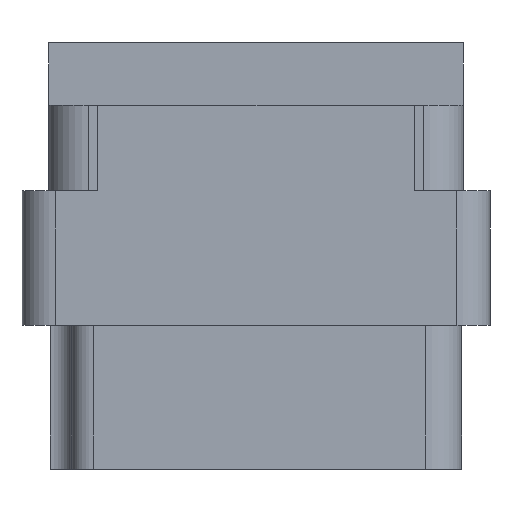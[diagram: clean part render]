
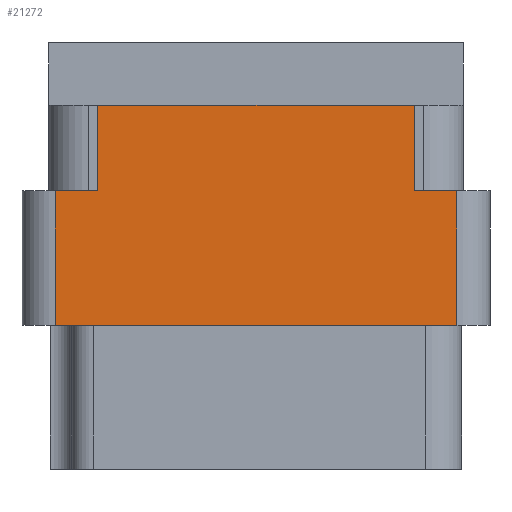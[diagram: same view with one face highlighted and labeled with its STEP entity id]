
A CAD part, left-side view. The second image highlights one B-rep face of the part: STEP entity #21272.
In plain terms, the highlighted planar face has unit normal (-1, 0, 0).
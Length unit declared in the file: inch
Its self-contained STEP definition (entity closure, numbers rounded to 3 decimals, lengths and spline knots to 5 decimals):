
#148 = LINE ( 'NONE', #6641, #24784 ) ;
#484 = CARTESIAN_POINT ( 'NONE',  ( -1., -0.296, -0.277 ) ) ;
#1525 = LINE ( 'NONE', #2006, #23892 ) ;
#2006 = CARTESIAN_POINT ( 'NONE',  ( -1., 0.376, -0.798 ) ) ;
#3123 = VECTOR ( 'NONE', #9455, 39.37008 ) ;
#3602 = ORIENTED_EDGE ( 'NONE', *, *, #24402, .T. ) ;
#3899 = CARTESIAN_POINT ( 'NONE',  ( -1., 0.438, -0.117 ) ) ;
#4356 = VERTEX_POINT ( 'NONE', #29186 ) ;
#5796 = LINE ( 'NONE', #8620, #27107 ) ;
#6131 = FACE_OUTER_BOUND ( 'NONE', #24997, .T. ) ;
#6449 = DIRECTION ( 'NONE',  ( 0., -1., 0. ) ) ;
#6541 = ORIENTED_EDGE ( 'NONE', *, *, #11253, .F. ) ;
#6623 = DIRECTION ( 'NONE',  ( 0., -1., 0. ) ) ;
#6641 = CARTESIAN_POINT ( 'NONE',  ( -1., 0., -0.277 ) ) ;
#6715 = EDGE_CURVE ( 'NONE', #22369, #12009, #7231, .T. ) ;
#6824 = DIRECTION ( 'NONE',  ( -1., 0., 0. ) ) ;
#7122 = VECTOR ( 'NONE', #14077, 39.37008 ) ;
#7231 = LINE ( 'NONE', #28528, #3123 ) ;
#8423 = CARTESIAN_POINT ( 'NONE',  ( -1., 0.376, -0.277 ) ) ;
#8446 = ORIENTED_EDGE ( 'NONE', *, *, #28309, .F. ) ;
#8620 = CARTESIAN_POINT ( 'NONE',  ( -1., 0., -0.529 ) ) ;
#8628 = ORIENTED_EDGE ( 'NONE', *, *, #17195, .T. ) ;
#8673 = CARTESIAN_POINT ( 'NONE',  ( -1., 0., -0.277 ) ) ;
#9052 = LINE ( 'NONE', #8673, #25108 ) ;
#9233 = DIRECTION ( 'NONE',  ( 0., 0., 1. ) ) ;
#9455 = DIRECTION ( 'NONE',  ( 0., 0., 1. ) ) ;
#10005 = ORIENTED_EDGE ( 'NONE', *, *, #29728, .F. ) ;
#10011 = VECTOR ( 'NONE', #21728, 39.37008 ) ;
#10602 = AXIS2_PLACEMENT_3D ( 'NONE', #21244, #6824, #9233 ) ;
#11157 = VERTEX_POINT ( 'NONE', #17635 ) ;
#11209 = DIRECTION ( 'NONE',  ( 0., 1., 0. ) ) ;
#11253 = EDGE_CURVE ( 'NONE', #19282, #28829, #148, .T. ) ;
#11858 = DIRECTION ( 'NONE',  ( 0., -1., 0. ) ) ;
#11996 = ORIENTED_EDGE ( 'NONE', *, *, #6715, .T. ) ;
#12009 = VERTEX_POINT ( 'NONE', #27760 ) ;
#12790 = CARTESIAN_POINT ( 'NONE',  ( -1., -0.376, -0.277 ) ) ;
#13379 = LINE ( 'NONE', #3899, #25667 ) ;
#14077 = DIRECTION ( 'NONE',  ( 0., 0., 1. ) ) ;
#17195 = EDGE_CURVE ( 'NONE', #4356, #26193, #20600, .T. ) ;
#17635 = CARTESIAN_POINT ( 'NONE',  ( -1., 0.296, -0.117 ) ) ;
#19282 = VERTEX_POINT ( 'NONE', #8423 ) ;
#19382 = EDGE_CURVE ( 'NONE', #11157, #12009, #13379, .T. ) ;
#20600 = LINE ( 'NONE', #21190, #7122 ) ;
#21128 = DIRECTION ( 'NONE',  ( 0., 0., -1. ) ) ;
#21190 = CARTESIAN_POINT ( 'NONE',  ( -1., -0.376, -0.798 ) ) ;
#21244 = CARTESIAN_POINT ( 'NONE',  ( -1., -0.438, -0.798 ) ) ;
#21272 = ADVANCED_FACE ( 'NONE', ( #6131 ), #25707, .T. ) ;
#21728 = DIRECTION ( 'NONE',  ( 0., 0., 1. ) ) ;
#22369 = VERTEX_POINT ( 'NONE', #484 ) ;
#23216 = EDGE_CURVE ( 'NONE', #22369, #26193, #9052, .T. ) ;
#23492 = LINE ( 'NONE', #24313, #10011 ) ;
#23892 = VECTOR ( 'NONE', #21128, 39.37008 ) ;
#24313 = CARTESIAN_POINT ( 'NONE',  ( -1., 0.296, -0.277 ) ) ;
#24402 = EDGE_CURVE ( 'NONE', #19282, #26761, #1525, .T. ) ;
#24784 = VECTOR ( 'NONE', #11858, 39.37008 ) ;
#24997 = EDGE_LOOP ( 'NONE', ( #6541, #3602, #10005, #8628, #25257, #11996, #27886, #8446 ) ) ;
#25108 = VECTOR ( 'NONE', #6449, 39.37008 ) ;
#25257 = ORIENTED_EDGE ( 'NONE', *, *, #23216, .F. ) ;
#25667 = VECTOR ( 'NONE', #6623, 39.37008 ) ;
#25707 = PLANE ( 'NONE',  #10602 ) ;
#26193 = VERTEX_POINT ( 'NONE', #12790 ) ;
#26761 = VERTEX_POINT ( 'NONE', #26833 ) ;
#26833 = CARTESIAN_POINT ( 'NONE',  ( -1., 0.376, -0.529 ) ) ;
#27107 = VECTOR ( 'NONE', #11209, 39.37008 ) ;
#27760 = CARTESIAN_POINT ( 'NONE',  ( -1., -0.296, -0.117 ) ) ;
#27886 = ORIENTED_EDGE ( 'NONE', *, *, #19382, .F. ) ;
#28309 = EDGE_CURVE ( 'NONE', #28829, #11157, #23492, .T. ) ;
#28528 = CARTESIAN_POINT ( 'NONE',  ( -1., -0.296, -0.277 ) ) ;
#28829 = VERTEX_POINT ( 'NONE', #30739 ) ;
#29186 = CARTESIAN_POINT ( 'NONE',  ( -1., -0.376, -0.529 ) ) ;
#29728 = EDGE_CURVE ( 'NONE', #4356, #26761, #5796, .T. ) ;
#30739 = CARTESIAN_POINT ( 'NONE',  ( -1., 0.296, -0.277 ) ) ;
